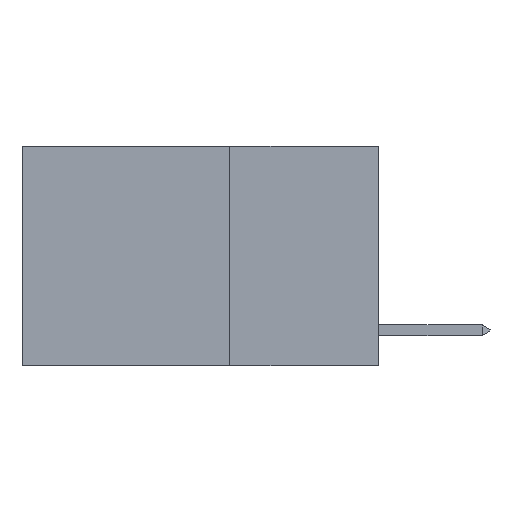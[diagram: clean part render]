
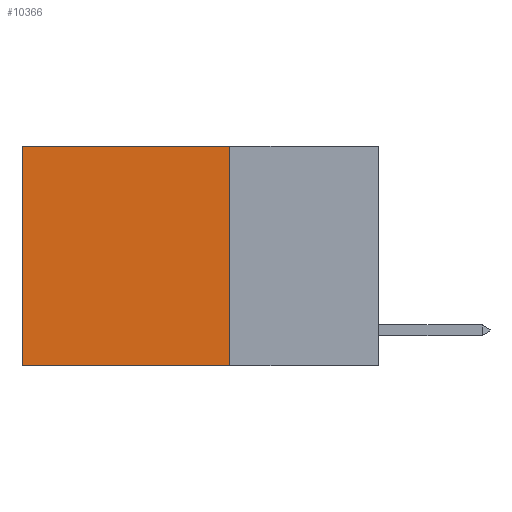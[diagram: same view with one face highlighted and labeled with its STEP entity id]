
A CAD part, left-side view. The second image highlights one B-rep face of the part: STEP entity #10366.
In plain terms, the highlighted planar face has unit normal (-1, 0, 0).
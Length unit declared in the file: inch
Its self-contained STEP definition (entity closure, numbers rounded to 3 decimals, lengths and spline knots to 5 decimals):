
#687 = VERTEX_POINT ( 'NONE', #1357 ) ;
#892 = DIRECTION ( 'NONE',  ( 0., 0., -1. ) ) ;
#1186 = EDGE_LOOP ( 'NONE', ( #8332, #26517, #23819, #8466 ) ) ;
#1357 = CARTESIAN_POINT ( 'NONE',  ( 0.2625, 0.25, -0.37 ) ) ;
#1577 = VECTOR ( 'NONE', #10376, 39.37008 ) ;
#1818 = DIRECTION ( 'NONE',  ( 0., 1., 0. ) ) ;
#2391 = FACE_OUTER_BOUND ( 'NONE', #1186, .T. ) ;
#2738 = LINE ( 'NONE', #14509, #24597 ) ;
#3221 = LINE ( 'NONE', #4625, #1577 ) ;
#3945 = DIRECTION ( 'NONE',  ( 0., 1., 0. ) ) ;
#4092 = CARTESIAN_POINT ( 'NONE',  ( 0.2625, 0.25, 0. ) ) ;
#4125 = EDGE_CURVE ( 'NONE', #12042, #687, #3221, .T. ) ;
#4625 = CARTESIAN_POINT ( 'NONE',  ( 0.2625, 0.25, 0. ) ) ;
#5599 = CARTESIAN_POINT ( 'NONE',  ( 0.2625, 0.6, 0. ) ) ;
#7153 = PLANE ( 'NONE',  #25734 ) ;
#8031 = DIRECTION ( 'NONE',  ( 0., 0., -1. ) ) ;
#8332 = ORIENTED_EDGE ( 'NONE', *, *, #24904, .T. ) ;
#8466 = ORIENTED_EDGE ( 'NONE', *, *, #18763, .T. ) ;
#8992 = EDGE_CURVE ( 'NONE', #687, #24448, #24024, .T. ) ;
#9187 = DIRECTION ( 'NONE',  ( 1., 0., 0. ) ) ;
#10366 = ADVANCED_FACE ( 'NONE', ( #2391 ), #7153, .F. ) ;
#10376 = DIRECTION ( 'NONE',  ( 0., 0., -1. ) ) ;
#12042 = VERTEX_POINT ( 'NONE', #4092 ) ;
#14509 = CARTESIAN_POINT ( 'NONE',  ( 0.2625, 0.25, 0. ) ) ;
#14934 = VERTEX_POINT ( 'NONE', #20048 ) ;
#15562 = LINE ( 'NONE', #5599, #19083 ) ;
#17256 = VECTOR ( 'NONE', #1818, 39.37008 ) ;
#18763 = EDGE_CURVE ( 'NONE', #12042, #14934, #2738, .T. ) ;
#19083 = VECTOR ( 'NONE', #8031, 39.37008 ) ;
#19664 = CARTESIAN_POINT ( 'NONE',  ( 0.2625, 0.6, -0.37 ) ) ;
#20048 = CARTESIAN_POINT ( 'NONE',  ( 0.2625, 0.6, 0. ) ) ;
#20567 = CARTESIAN_POINT ( 'NONE',  ( 0.2625, 0.25, -0.37 ) ) ;
#23819 = ORIENTED_EDGE ( 'NONE', *, *, #4125, .F. ) ;
#23825 = CARTESIAN_POINT ( 'NONE',  ( 0.2625, 0.25, 0. ) ) ;
#24024 = LINE ( 'NONE', #20567, #17256 ) ;
#24448 = VERTEX_POINT ( 'NONE', #19664 ) ;
#24597 = VECTOR ( 'NONE', #3945, 39.37008 ) ;
#24904 = EDGE_CURVE ( 'NONE', #14934, #24448, #15562, .T. ) ;
#25734 = AXIS2_PLACEMENT_3D ( 'NONE', #23825, #9187, #892 ) ;
#26517 = ORIENTED_EDGE ( 'NONE', *, *, #8992, .F. ) ;
